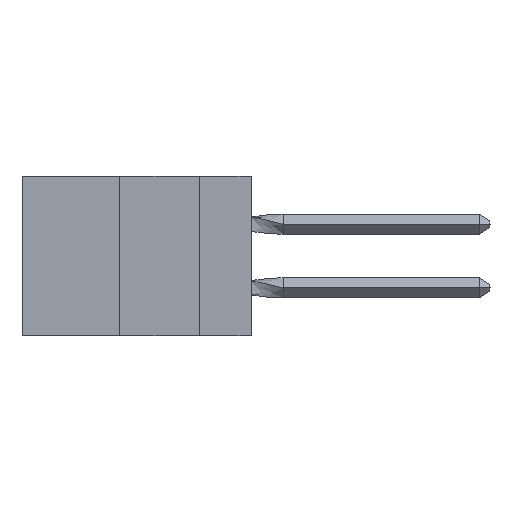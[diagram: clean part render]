
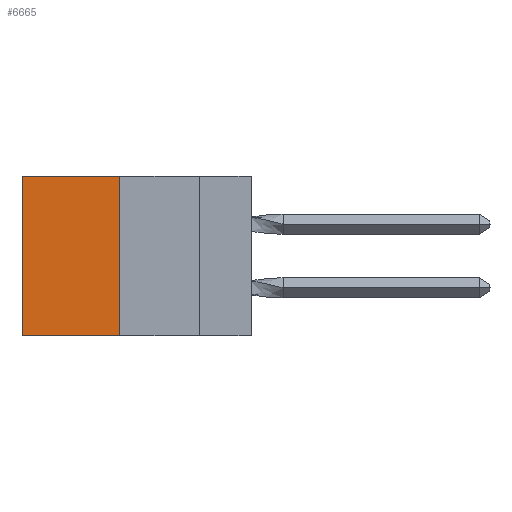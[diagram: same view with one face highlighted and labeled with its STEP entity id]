
A CAD part, left-side view. The second image highlights one B-rep face of the part: STEP entity #6665.
In plain terms, the highlighted planar face has unit normal (-1, 0, 0).
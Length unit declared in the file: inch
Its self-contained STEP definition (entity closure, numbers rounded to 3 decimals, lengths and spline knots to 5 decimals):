
#2143 = PLANE ( 'NONE',  #15352 ) ;
#2307 = DIRECTION ( 'NONE',  ( 0., 1., 0. ) ) ;
#2372 = VECTOR ( 'NONE', #19015, 39.37008 ) ;
#3923 = DIRECTION ( 'NONE',  ( 0., 0., -1. ) ) ;
#4859 = FACE_OUTER_BOUND ( 'NONE', #19802, .T. ) ;
#6654 = VERTEX_POINT ( 'NONE', #37429 ) ;
#6665 = ADVANCED_FACE ( 'NONE', ( #4859 ), #2143, .F. ) ;
#7094 = VERTEX_POINT ( 'NONE', #36603 ) ;
#9792 = CARTESIAN_POINT ( 'NONE',  ( 0.305, 0.72, 0. ) ) ;
#15352 = AXIS2_PLACEMENT_3D ( 'NONE', #22293, #25364, #3923 ) ;
#15888 = CARTESIAN_POINT ( 'NONE',  ( 0.305, 0.413, -0.5 ) ) ;
#16085 = EDGE_CURVE ( 'NONE', #7094, #6654, #39324, .T. ) ;
#16240 = LINE ( 'NONE', #27732, #40680 ) ;
#19015 = DIRECTION ( 'NONE',  ( 0., 0., -1. ) ) ;
#19802 = EDGE_LOOP ( 'NONE', ( #29476, #20541, #30679, #24871 ) ) ;
#20541 = ORIENTED_EDGE ( 'NONE', *, *, #16085, .F. ) ;
#21239 = CARTESIAN_POINT ( 'NONE',  ( 0.305, 0.413, -0.5 ) ) ;
#21297 = LINE ( 'NONE', #15888, #2372 ) ;
#21738 = LINE ( 'NONE', #25037, #40193 ) ;
#22293 = CARTESIAN_POINT ( 'NONE',  ( 0.305, 0.413, -0.5 ) ) ;
#24531 = DIRECTION ( 'NONE',  ( 0., 1., 0. ) ) ;
#24871 = ORIENTED_EDGE ( 'NONE', *, *, #30499, .T. ) ;
#25037 = CARTESIAN_POINT ( 'NONE',  ( 0.305, 0.72, -0.5 ) ) ;
#25364 = DIRECTION ( 'NONE',  ( 1., 0., 0. ) ) ;
#25546 = EDGE_CURVE ( 'NONE', #29146, #6654, #21738, .T. ) ;
#27732 = CARTESIAN_POINT ( 'NONE',  ( 0.305, 0.413, 0. ) ) ;
#29146 = VERTEX_POINT ( 'NONE', #9792 ) ;
#29476 = ORIENTED_EDGE ( 'NONE', *, *, #25546, .T. ) ;
#29810 = VERTEX_POINT ( 'NONE', #41321 ) ;
#30499 = EDGE_CURVE ( 'NONE', #29810, #29146, #16240, .T. ) ;
#30679 = ORIENTED_EDGE ( 'NONE', *, *, #38474, .F. ) ;
#34343 = VECTOR ( 'NONE', #2307, 39.37008 ) ;
#36603 = CARTESIAN_POINT ( 'NONE',  ( 0.305, 0.413, -0.5 ) ) ;
#37429 = CARTESIAN_POINT ( 'NONE',  ( 0.305, 0.72, -0.5 ) ) ;
#38474 = EDGE_CURVE ( 'NONE', #29810, #7094, #21297, .T. ) ;
#39324 = LINE ( 'NONE', #21239, #34343 ) ;
#40193 = VECTOR ( 'NONE', #40516, 39.37008 ) ;
#40516 = DIRECTION ( 'NONE',  ( 0., 0., -1. ) ) ;
#40680 = VECTOR ( 'NONE', #24531, 39.37008 ) ;
#41321 = CARTESIAN_POINT ( 'NONE',  ( 0.305, 0.413, 0. ) ) ;
